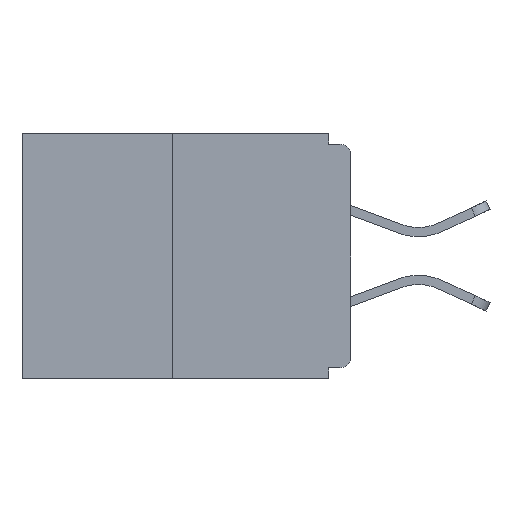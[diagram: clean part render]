
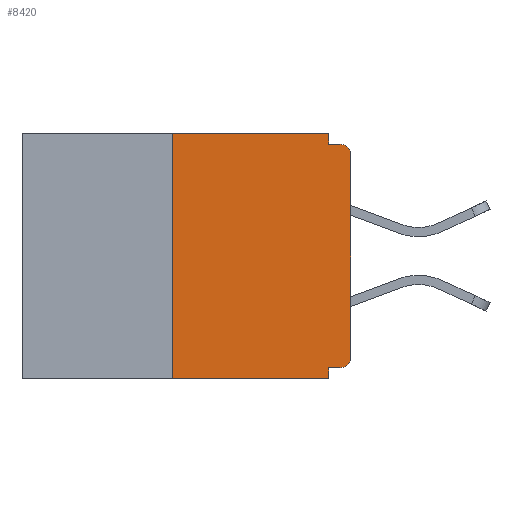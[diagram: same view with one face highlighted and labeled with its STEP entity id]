
A CAD part, left-side view. The second image highlights one B-rep face of the part: STEP entity #8420.
In plain terms, the highlighted planar face has unit normal (-1, 0, 0).
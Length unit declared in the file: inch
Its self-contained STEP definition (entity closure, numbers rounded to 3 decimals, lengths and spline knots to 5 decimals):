
#186 = VERTEX_POINT ( 'NONE', #3896 ) ;
#374 = CARTESIAN_POINT ( 'NONE',  ( 0., 0.031, -0.328 ) ) ;
#539 = EDGE_LOOP ( 'NONE', ( #12361, #8967, #8840, #7408, #5512, #4658, #4108, #10308, #866, #3047 ) ) ;
#702 = CARTESIAN_POINT ( 'NONE',  ( 0., 0., -0.313 ) ) ;
#866 = ORIENTED_EDGE ( 'NONE', *, *, #12743, .F. ) ;
#950 = VECTOR ( 'NONE', #11382, 39.37008 ) ;
#984 = CARTESIAN_POINT ( 'NONE',  ( 0., 0., 0. ) ) ;
#1429 = DIRECTION ( 'NONE',  ( 0., 0., -1. ) ) ;
#1439 = VERTEX_POINT ( 'NONE', #3816 ) ;
#1529 = LINE ( 'NONE', #6682, #10930 ) ;
#1548 = CARTESIAN_POINT ( 'NONE',  ( 0., 0., -0.015 ) ) ;
#1971 = LINE ( 'NONE', #5925, #8324 ) ;
#2011 = VERTEX_POINT ( 'NONE', #702 ) ;
#2110 = EDGE_CURVE ( 'NONE', #1439, #8011, #6706, .T. ) ;
#2196 = VERTEX_POINT ( 'NONE', #8064 ) ;
#2614 = AXIS2_PLACEMENT_3D ( 'NONE', #4606, #5438, #1429 ) ;
#2951 = VERTEX_POINT ( 'NONE', #9399 ) ;
#2964 = VERTEX_POINT ( 'NONE', #12531 ) ;
#3047 = ORIENTED_EDGE ( 'NONE', *, *, #7742, .F. ) ;
#3305 = VECTOR ( 'NONE', #5891, 39.37008 ) ;
#3816 = CARTESIAN_POINT ( 'NONE',  ( 0., 0.25, 0. ) ) ;
#3896 = CARTESIAN_POINT ( 'NONE',  ( 0., 0.031, -0.015 ) ) ;
#3991 = DIRECTION ( 'NONE',  ( -1., 0., 0. ) ) ;
#4070 = VECTOR ( 'NONE', #9836, 39.37008 ) ;
#4108 = ORIENTED_EDGE ( 'NONE', *, *, #7793, .T. ) ;
#4163 = EDGE_CURVE ( 'NONE', #11980, #12214, #5859, .T. ) ;
#4209 = EDGE_CURVE ( 'NONE', #2196, #2964, #8013, .T. ) ;
#4427 = EDGE_CURVE ( 'NONE', #8368, #11980, #1971, .T. ) ;
#4468 = FACE_OUTER_BOUND ( 'NONE', #539, .T. ) ;
#4606 = CARTESIAN_POINT ( 'NONE',  ( 0., 0.015, -0.03 ) ) ;
#4658 = ORIENTED_EDGE ( 'NONE', *, *, #8416, .T. ) ;
#5168 = CARTESIAN_POINT ( 'NONE',  ( 0., 0.46, -0.343 ) ) ;
#5409 = AXIS2_PLACEMENT_3D ( 'NONE', #10236, #3991, #12290 ) ;
#5438 = DIRECTION ( 'NONE',  ( -1., 0., 0. ) ) ;
#5512 = ORIENTED_EDGE ( 'NONE', *, *, #4427, .F. ) ;
#5516 = LINE ( 'NONE', #1548, #4070 ) ;
#5603 = CARTESIAN_POINT ( 'NONE',  ( 0., 0.031, -0.343 ) ) ;
#5635 = LINE ( 'NONE', #5168, #6297 ) ;
#5823 = CARTESIAN_POINT ( 'NONE',  ( 0., 0.031, 0. ) ) ;
#5859 = LINE ( 'NONE', #5603, #7355 ) ;
#5891 = DIRECTION ( 'NONE',  ( 0., -1., 0. ) ) ;
#5925 = CARTESIAN_POINT ( 'NONE',  ( 0., 0., -0.328 ) ) ;
#5928 = CARTESIAN_POINT ( 'NONE',  ( 0., 0.031, 0. ) ) ;
#6035 = DIRECTION ( 'NONE',  ( 1., 0., 0. ) ) ;
#6288 = LINE ( 'NONE', #984, #950 ) ;
#6297 = VECTOR ( 'NONE', #12502, 39.37008 ) ;
#6423 = CIRCLE ( 'NONE', #5409, 0.015 ) ;
#6682 = CARTESIAN_POINT ( 'NONE',  ( 0., 0.25, 0. ) ) ;
#6706 = LINE ( 'NONE', #10040, #3305 ) ;
#7092 = PLANE ( 'NONE',  #11456 ) ;
#7331 = EDGE_CURVE ( 'NONE', #2951, #12214, #5635, .T. ) ;
#7355 = VECTOR ( 'NONE', #11777, 39.37008 ) ;
#7408 = ORIENTED_EDGE ( 'NONE', *, *, #4163, .F. ) ;
#7742 = EDGE_CURVE ( 'NONE', #8011, #186, #9057, .T. ) ;
#7793 = EDGE_CURVE ( 'NONE', #2011, #2196, #6288, .T. ) ;
#8011 = VERTEX_POINT ( 'NONE', #5928 ) ;
#8013 = CIRCLE ( 'NONE', #2614, 0.015 ) ;
#8064 = CARTESIAN_POINT ( 'NONE',  ( 0., 0., -0.03 ) ) ;
#8324 = VECTOR ( 'NONE', #13259, 39.37008 ) ;
#8368 = VERTEX_POINT ( 'NONE', #11001 ) ;
#8416 = EDGE_CURVE ( 'NONE', #8368, #2011, #6423, .T. ) ;
#8420 = ADVANCED_FACE ( 'NONE', ( #4468 ), #7092, .F. ) ;
#8840 = ORIENTED_EDGE ( 'NONE', *, *, #7331, .T. ) ;
#8967 = ORIENTED_EDGE ( 'NONE', *, *, #10949, .F. ) ;
#9057 = LINE ( 'NONE', #5823, #13286 ) ;
#9399 = CARTESIAN_POINT ( 'NONE',  ( 0., 0.25, -0.343 ) ) ;
#9836 = DIRECTION ( 'NONE',  ( 0., -1., 0. ) ) ;
#10040 = CARTESIAN_POINT ( 'NONE',  ( 0., 0.46, 0. ) ) ;
#10236 = CARTESIAN_POINT ( 'NONE',  ( 0., 0.015, -0.313 ) ) ;
#10308 = ORIENTED_EDGE ( 'NONE', *, *, #4209, .T. ) ;
#10868 = DIRECTION ( 'NONE',  ( 0., 0., 1. ) ) ;
#10930 = VECTOR ( 'NONE', #10868, 39.37008 ) ;
#10949 = EDGE_CURVE ( 'NONE', #2951, #1439, #1529, .T. ) ;
#11001 = CARTESIAN_POINT ( 'NONE',  ( 0., 0.015, -0.328 ) ) ;
#11045 = CARTESIAN_POINT ( 'NONE',  ( 0., 0.031, -0.343 ) ) ;
#11285 = CARTESIAN_POINT ( 'NONE',  ( 0., 0.46, 0. ) ) ;
#11331 = DIRECTION ( 'NONE',  ( 0., 0., -1. ) ) ;
#11382 = DIRECTION ( 'NONE',  ( 0., 0., 1. ) ) ;
#11456 = AXIS2_PLACEMENT_3D ( 'NONE', #11285, #6035, #11331 ) ;
#11777 = DIRECTION ( 'NONE',  ( 0., 0., -1. ) ) ;
#11980 = VERTEX_POINT ( 'NONE', #374 ) ;
#12214 = VERTEX_POINT ( 'NONE', #11045 ) ;
#12290 = DIRECTION ( 'NONE',  ( 0., 0., -1. ) ) ;
#12361 = ORIENTED_EDGE ( 'NONE', *, *, #2110, .F. ) ;
#12502 = DIRECTION ( 'NONE',  ( 0., -1., 0. ) ) ;
#12531 = CARTESIAN_POINT ( 'NONE',  ( 0., 0.015, -0.015 ) ) ;
#12743 = EDGE_CURVE ( 'NONE', #186, #2964, #5516, .T. ) ;
#13114 = DIRECTION ( 'NONE',  ( 0., 0., -1. ) ) ;
#13259 = DIRECTION ( 'NONE',  ( 0., 1., 0. ) ) ;
#13286 = VECTOR ( 'NONE', #13114, 39.37008 ) ;
